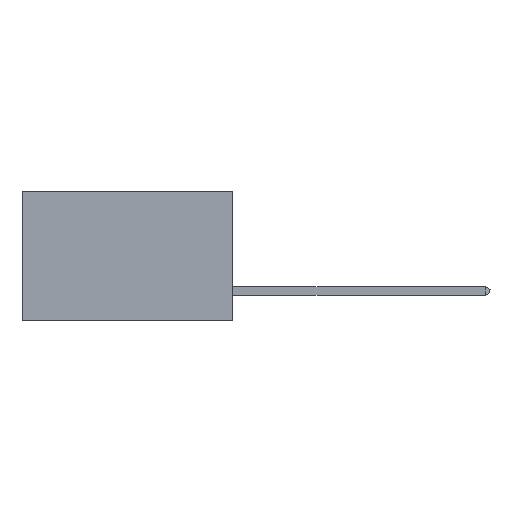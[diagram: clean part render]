
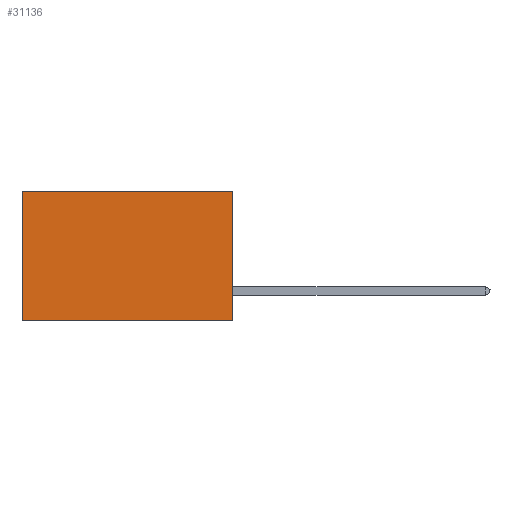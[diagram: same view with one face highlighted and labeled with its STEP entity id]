
A CAD part, left-side view. The second image highlights one B-rep face of the part: STEP entity #31136.
In plain terms, the highlighted planar face has unit normal (-1, 0, 0).
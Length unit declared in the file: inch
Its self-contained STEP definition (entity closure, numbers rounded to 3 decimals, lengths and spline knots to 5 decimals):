
#812 = EDGE_CURVE ( 'NONE', #9056, #2239, #20463, .T. ) ;
#1277 = VECTOR ( 'NONE', #3297, 39.37008 ) ;
#2239 = VERTEX_POINT ( 'NONE', #9658 ) ;
#2975 = ORIENTED_EDGE ( 'NONE', *, *, #21231, .T. ) ;
#3297 = DIRECTION ( 'NONE',  ( 0., 1., 0. ) ) ;
#4261 = AXIS2_PLACEMENT_3D ( 'NONE', #14178, #4846, #14326 ) ;
#4846 = DIRECTION ( 'NONE',  ( 1., 0., 0. ) ) ;
#6663 = DIRECTION ( 'NONE',  ( 0., 1., 0. ) ) ;
#6870 = EDGE_CURVE ( 'NONE', #2239, #36386, #35766, .T. ) ;
#9007 = CARTESIAN_POINT ( 'NONE',  ( 0.2875, 0., 0. ) ) ;
#9056 = VERTEX_POINT ( 'NONE', #37623 ) ;
#9658 = CARTESIAN_POINT ( 'NONE',  ( 0.2875, 0., -0.37 ) ) ;
#11350 = CARTESIAN_POINT ( 'NONE',  ( 0.2875, 0.6, 0. ) ) ;
#13787 = VECTOR ( 'NONE', #20785, 39.37008 ) ;
#14178 = CARTESIAN_POINT ( 'NONE',  ( 0.2875, 0., 0. ) ) ;
#14326 = DIRECTION ( 'NONE',  ( 0., 0., -1. ) ) ;
#14926 = CARTESIAN_POINT ( 'NONE',  ( 0.2875, 0.6, 0. ) ) ;
#15315 = CARTESIAN_POINT ( 'NONE',  ( 0.2875, 0., 0. ) ) ;
#15772 = CARTESIAN_POINT ( 'NONE',  ( 0.2875, 0.6, -0.37 ) ) ;
#18022 = VECTOR ( 'NONE', #19559, 39.37008 ) ;
#19559 = DIRECTION ( 'NONE',  ( 0., 0., -1. ) ) ;
#20463 = LINE ( 'NONE', #9007, #18022 ) ;
#20785 = DIRECTION ( 'NONE',  ( 0., 0., -1. ) ) ;
#21231 = EDGE_CURVE ( 'NONE', #9056, #24266, #34723, .T. ) ;
#22076 = ORIENTED_EDGE ( 'NONE', *, *, #6870, .F. ) ;
#22118 = LINE ( 'NONE', #11350, #13787 ) ;
#24266 = VERTEX_POINT ( 'NONE', #14926 ) ;
#24328 = ORIENTED_EDGE ( 'NONE', *, *, #812, .F. ) ;
#24816 = EDGE_CURVE ( 'NONE', #24266, #36386, #22118, .T. ) ;
#27207 = PLANE ( 'NONE',  #4261 ) ;
#29145 = FACE_OUTER_BOUND ( 'NONE', #39449, .T. ) ;
#29862 = VECTOR ( 'NONE', #6663, 39.37008 ) ;
#31136 = ADVANCED_FACE ( 'NONE', ( #29145 ), #27207, .F. ) ;
#34444 = CARTESIAN_POINT ( 'NONE',  ( 0.2875, 0., -0.37 ) ) ;
#34723 = LINE ( 'NONE', #15315, #1277 ) ;
#35766 = LINE ( 'NONE', #34444, #29862 ) ;
#36386 = VERTEX_POINT ( 'NONE', #15772 ) ;
#37623 = CARTESIAN_POINT ( 'NONE',  ( 0.2875, 0., 0. ) ) ;
#38878 = ORIENTED_EDGE ( 'NONE', *, *, #24816, .T. ) ;
#39449 = EDGE_LOOP ( 'NONE', ( #38878, #22076, #24328, #2975 ) ) ;
